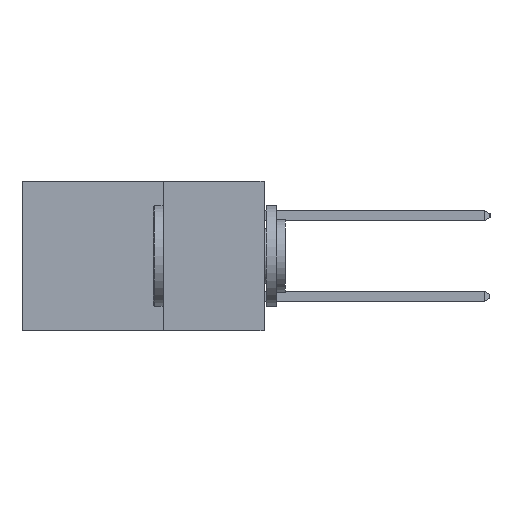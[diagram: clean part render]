
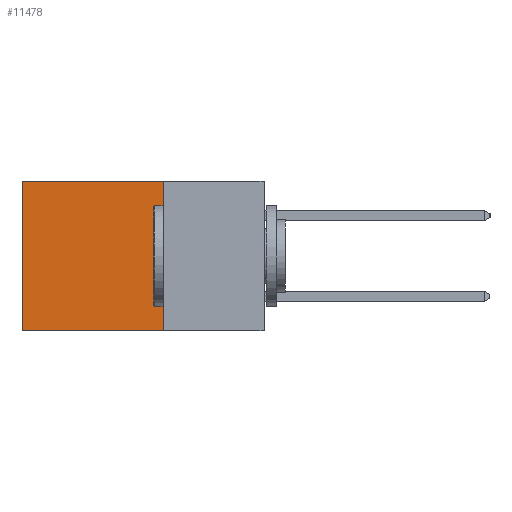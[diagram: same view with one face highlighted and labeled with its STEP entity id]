
A CAD part, left-side view. The second image highlights one B-rep face of the part: STEP entity #11478.
In plain terms, the highlighted planar face has unit normal (-1, 0, 0).
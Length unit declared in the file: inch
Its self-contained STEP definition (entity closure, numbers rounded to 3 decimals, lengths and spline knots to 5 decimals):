
#243 = FACE_OUTER_BOUND ( 'NONE', #5056, .T. ) ;
#1982 = ORIENTED_EDGE ( 'NONE', *, *, #21074, .F. ) ;
#2182 = VERTEX_POINT ( 'NONE', #14555 ) ;
#2377 = CARTESIAN_POINT ( 'NONE',  ( 0.2615, 0.6, -0.37 ) ) ;
#3111 = CARTESIAN_POINT ( 'NONE',  ( 0.2615, 0.25, 0. ) ) ;
#3880 = VECTOR ( 'NONE', #15802, 39.37008 ) ;
#3916 = AXIS2_PLACEMENT_3D ( 'NONE', #8979, #23563, #22116 ) ;
#4016 = DIRECTION ( 'NONE',  ( 0., 1., 0. ) ) ;
#4894 = EDGE_CURVE ( 'NONE', #2182, #21393, #7492, .T. ) ;
#5056 = EDGE_LOOP ( 'NONE', ( #19985, #10618, #1982, #21139 ) ) ;
#5136 = CARTESIAN_POINT ( 'NONE',  ( 0.2615, 0.25, -0.37 ) ) ;
#5872 = VECTOR ( 'NONE', #13038, 39.37008 ) ;
#7061 = DIRECTION ( 'NONE',  ( 0., 0., -1. ) ) ;
#7341 = CARTESIAN_POINT ( 'NONE',  ( 0.2615, 0.6, 0. ) ) ;
#7492 = LINE ( 'NONE', #12996, #18687 ) ;
#8412 = VERTEX_POINT ( 'NONE', #7341 ) ;
#8979 = CARTESIAN_POINT ( 'NONE',  ( 0.2615, 0.25, -0.37 ) ) ;
#9336 = CARTESIAN_POINT ( 'NONE',  ( 0.2615, 0.6, -0.37 ) ) ;
#9944 = EDGE_CURVE ( 'NONE', #15717, #8412, #12202, .T. ) ;
#10618 = ORIENTED_EDGE ( 'NONE', *, *, #4894, .F. ) ;
#11378 = CARTESIAN_POINT ( 'NONE',  ( 0.2615, 0.25, 0. ) ) ;
#11478 = ADVANCED_FACE ( 'NONE', ( #243 ), #14829, .F. ) ;
#12202 = LINE ( 'NONE', #3111, #3880 ) ;
#12443 = LINE ( 'NONE', #5136, #22922 ) ;
#12808 = EDGE_CURVE ( 'NONE', #8412, #21393, #18643, .T. ) ;
#12996 = CARTESIAN_POINT ( 'NONE',  ( 0.2615, 0.25, -0.37 ) ) ;
#13038 = DIRECTION ( 'NONE',  ( 0., 0., -1. ) ) ;
#14555 = CARTESIAN_POINT ( 'NONE',  ( 0.2615, 0.25, -0.37 ) ) ;
#14829 = PLANE ( 'NONE',  #3916 ) ;
#15717 = VERTEX_POINT ( 'NONE', #11378 ) ;
#15802 = DIRECTION ( 'NONE',  ( 0., 1., 0. ) ) ;
#18643 = LINE ( 'NONE', #9336, #5872 ) ;
#18687 = VECTOR ( 'NONE', #4016, 39.37008 ) ;
#19985 = ORIENTED_EDGE ( 'NONE', *, *, #12808, .T. ) ;
#21074 = EDGE_CURVE ( 'NONE', #15717, #2182, #12443, .T. ) ;
#21139 = ORIENTED_EDGE ( 'NONE', *, *, #9944, .T. ) ;
#21393 = VERTEX_POINT ( 'NONE', #2377 ) ;
#22116 = DIRECTION ( 'NONE',  ( 0., 0., -1. ) ) ;
#22922 = VECTOR ( 'NONE', #7061, 39.37008 ) ;
#23563 = DIRECTION ( 'NONE',  ( 1., 0., 0. ) ) ;
